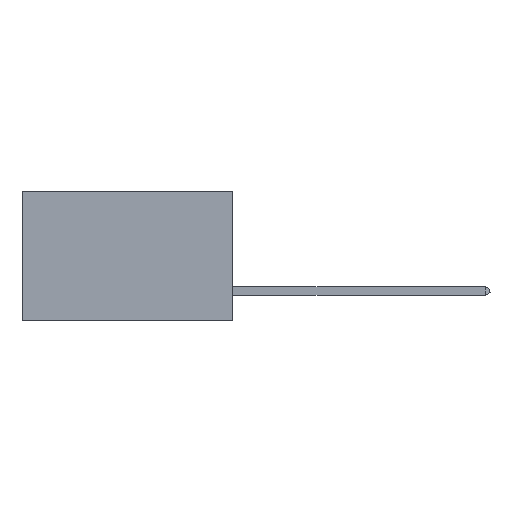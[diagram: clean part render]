
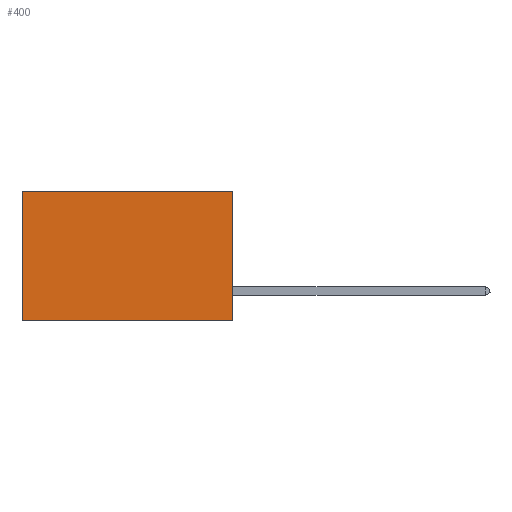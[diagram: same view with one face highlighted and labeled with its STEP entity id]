
A CAD part, left-side view. The second image highlights one B-rep face of the part: STEP entity #400.
In plain terms, the highlighted planar face has unit normal (-1, 0, 0).
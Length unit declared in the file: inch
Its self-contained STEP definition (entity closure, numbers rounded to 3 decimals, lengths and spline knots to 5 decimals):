
#102 = PLANE ( 'NONE',  #4672 ) ;
#400 = ADVANCED_FACE ( 'NONE', ( #8593 ), #102, .F. ) ;
#754 = ORIENTED_EDGE ( 'NONE', *, *, #9647, .F. ) ;
#941 = VERTEX_POINT ( 'NONE', #9370 ) ;
#1563 = CARTESIAN_POINT ( 'NONE',  ( 0.2875, 0., 0. ) ) ;
#1667 = DIRECTION ( 'NONE',  ( 0., 1., 0. ) ) ;
#1802 = CARTESIAN_POINT ( 'NONE',  ( 0.2875, 0., 0. ) ) ;
#1850 = DIRECTION ( 'NONE',  ( 0., 1., 0. ) ) ;
#2730 = ORIENTED_EDGE ( 'NONE', *, *, #11180, .T. ) ;
#3744 = CARTESIAN_POINT ( 'NONE',  ( 0.2875, 0., 0. ) ) ;
#3858 = LINE ( 'NONE', #6215, #11829 ) ;
#4127 = LINE ( 'NONE', #1802, #9758 ) ;
#4557 = VERTEX_POINT ( 'NONE', #5667 ) ;
#4672 = AXIS2_PLACEMENT_3D ( 'NONE', #3744, #8722, #10659 ) ;
#4971 = ORIENTED_EDGE ( 'NONE', *, *, #9506, .F. ) ;
#5009 = ORIENTED_EDGE ( 'NONE', *, *, #6198, .T. ) ;
#5066 = VECTOR ( 'NONE', #1667, 39.37008 ) ;
#5493 = VERTEX_POINT ( 'NONE', #1563 ) ;
#5508 = CARTESIAN_POINT ( 'NONE',  ( 0.2875, 0., 0. ) ) ;
#5667 = CARTESIAN_POINT ( 'NONE',  ( 0.2875, 0.6, -0.37 ) ) ;
#6198 = EDGE_CURVE ( 'NONE', #5493, #941, #4127, .T. ) ;
#6215 = CARTESIAN_POINT ( 'NONE',  ( 0.2875, 0.6, 0. ) ) ;
#8355 = LINE ( 'NONE', #5508, #9116 ) ;
#8440 = VERTEX_POINT ( 'NONE', #10727 ) ;
#8593 = FACE_OUTER_BOUND ( 'NONE', #10769, .T. ) ;
#8722 = DIRECTION ( 'NONE',  ( 1., 0., 0. ) ) ;
#9116 = VECTOR ( 'NONE', #11059, 39.37008 ) ;
#9308 = CARTESIAN_POINT ( 'NONE',  ( 0.2875, 0., -0.37 ) ) ;
#9370 = CARTESIAN_POINT ( 'NONE',  ( 0.2875, 0.6, 0. ) ) ;
#9506 = EDGE_CURVE ( 'NONE', #5493, #8440, #8355, .T. ) ;
#9647 = EDGE_CURVE ( 'NONE', #8440, #4557, #10386, .T. ) ;
#9758 = VECTOR ( 'NONE', #1850, 39.37008 ) ;
#10386 = LINE ( 'NONE', #9308, #5066 ) ;
#10659 = DIRECTION ( 'NONE',  ( 0., 0., -1. ) ) ;
#10727 = CARTESIAN_POINT ( 'NONE',  ( 0.2875, 0., -0.37 ) ) ;
#10769 = EDGE_LOOP ( 'NONE', ( #2730, #754, #4971, #5009 ) ) ;
#11059 = DIRECTION ( 'NONE',  ( 0., 0., -1. ) ) ;
#11180 = EDGE_CURVE ( 'NONE', #941, #4557, #3858, .T. ) ;
#11829 = VECTOR ( 'NONE', #11864, 39.37008 ) ;
#11864 = DIRECTION ( 'NONE',  ( 0., 0., -1. ) ) ;
